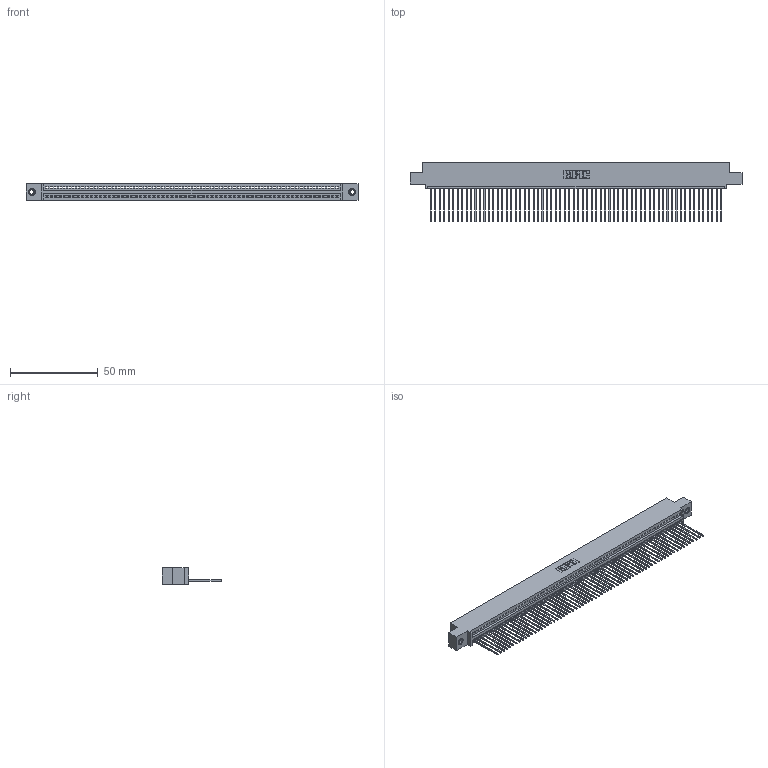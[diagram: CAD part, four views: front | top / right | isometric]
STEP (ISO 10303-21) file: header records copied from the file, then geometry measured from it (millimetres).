
FILE_DESCRIPTION (( 'STEP AP203' ), '1' );
FILE_NAME ('345-066-541-407.STEP', '2019-10-11T22:01:57', ( '' ), ( '' ), 'SwSTEP 2.0', 'SolidWorks 2016', '' );
FILE_SCHEMA (( 'CONFIG_CONTROL_DESIGN' ));
Length unit declared in the file: inch
Products named in the file (4): 345-292-001_345-293-141; 345-066-541-407; 345-250-001_345-250-005-103; 345 Part_0.110 Offset - 0.156 Dia-TI
Assembly tree (69 placements, depth 2):
  345-066-541-407
    345 Part_0.110 Offset - 0.156 Dia-TI
    345-292-001_345-293-141  x66
    345-250-001_345-250-005-103  x2
Bounding box: 188.85 x 33.96 x 9.4 mm (x, y, z)
Volume: 18264.6 mm3; surface area: 25994.1 mm2
Topology: 69 solids, 69 shells, 4018 faces, 12105 edges, 7974 vertices
Faces by surface type: plane 2756, cylinder 1246, cone 12, torus 4
Entity records: 47778 total; most frequent: CARTESIAN_POINT 8257, ORIENTED_EDGE 8250, DIRECTION 7203, EDGE_CURVE 4125, VECTOR 3709, LINE 3709, VERTEX_POINT 2744, AXIS2_PLACEMENT_3D 1747
